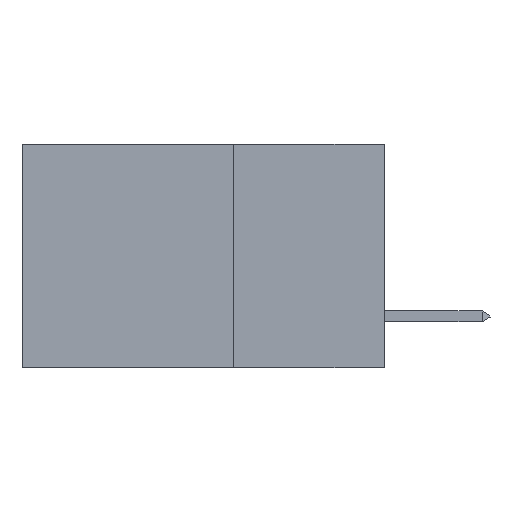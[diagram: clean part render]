
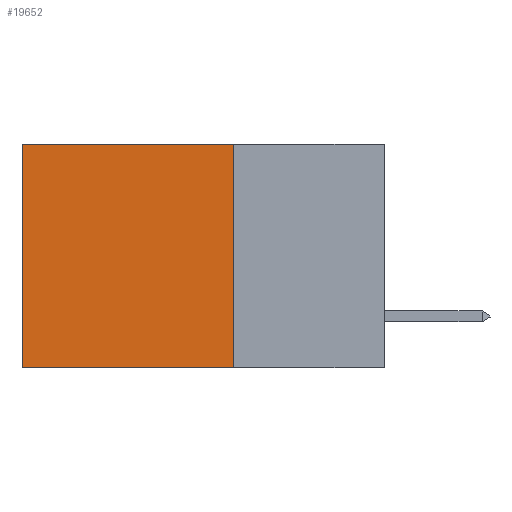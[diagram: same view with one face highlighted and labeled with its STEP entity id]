
A CAD part, left-side view. The second image highlights one B-rep face of the part: STEP entity #19652.
In plain terms, the highlighted planar face has unit normal (-1, 0, 0).
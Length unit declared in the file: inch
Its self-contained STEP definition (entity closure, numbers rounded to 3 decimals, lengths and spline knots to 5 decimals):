
#3214 = CARTESIAN_POINT ( 'NONE',  ( 0.2875, 0.25, 0. ) ) ;
#3326 = AXIS2_PLACEMENT_3D ( 'NONE', #8583, #22434, #37342 ) ;
#5509 = CARTESIAN_POINT ( 'NONE',  ( 0.2875, 0.25, -0.37 ) ) ;
#5762 = EDGE_CURVE ( 'NONE', #29457, #33184, #31142, .T. ) ;
#8160 = EDGE_CURVE ( 'NONE', #30288, #41633, #34900, .T. ) ;
#8583 = CARTESIAN_POINT ( 'NONE',  ( 0.2875, 0.25, 0. ) ) ;
#8875 = CARTESIAN_POINT ( 'NONE',  ( 0.2875, 0.25, 0. ) ) ;
#9150 = DIRECTION ( 'NONE',  ( 0., 1., 0. ) ) ;
#11128 = PLANE ( 'NONE',  #3326 ) ;
#11969 = LINE ( 'NONE', #22813, #42398 ) ;
#16475 = VECTOR ( 'NONE', #26170, 39.37008 ) ;
#19652 = ADVANCED_FACE ( 'NONE', ( #25178 ), #11128, .F. ) ;
#20322 = VECTOR ( 'NONE', #42332, 39.37008 ) ;
#20536 = CARTESIAN_POINT ( 'NONE',  ( 0.2875, 0.6, 0. ) ) ;
#21779 = ORIENTED_EDGE ( 'NONE', *, *, #8160, .F. ) ;
#22434 = DIRECTION ( 'NONE',  ( 1., 0., 0. ) ) ;
#22813 = CARTESIAN_POINT ( 'NONE',  ( 0.2875, 0.25, 0. ) ) ;
#25178 = FACE_OUTER_BOUND ( 'NONE', #35879, .T. ) ;
#25345 = VECTOR ( 'NONE', #9150, 39.37008 ) ;
#26170 = DIRECTION ( 'NONE',  ( 0., 1., 0. ) ) ;
#28706 = EDGE_CURVE ( 'NONE', #33184, #41633, #33818, .T. ) ;
#29457 = VERTEX_POINT ( 'NONE', #3214 ) ;
#30288 = VERTEX_POINT ( 'NONE', #37762 ) ;
#31142 = LINE ( 'NONE', #8875, #16475 ) ;
#33184 = VERTEX_POINT ( 'NONE', #36288 ) ;
#33818 = LINE ( 'NONE', #20536, #20322 ) ;
#34900 = LINE ( 'NONE', #5509, #25345 ) ;
#35879 = EDGE_LOOP ( 'NONE', ( #36474, #21779, #41128, #40969 ) ) ;
#36288 = CARTESIAN_POINT ( 'NONE',  ( 0.2875, 0.6, 0. ) ) ;
#36474 = ORIENTED_EDGE ( 'NONE', *, *, #28706, .T. ) ;
#37342 = DIRECTION ( 'NONE',  ( 0., 0., -1. ) ) ;
#37393 = DIRECTION ( 'NONE',  ( 0., 0., -1. ) ) ;
#37762 = CARTESIAN_POINT ( 'NONE',  ( 0.2875, 0.25, -0.37 ) ) ;
#40969 = ORIENTED_EDGE ( 'NONE', *, *, #5762, .T. ) ;
#41128 = ORIENTED_EDGE ( 'NONE', *, *, #42688, .F. ) ;
#41633 = VERTEX_POINT ( 'NONE', #45690 ) ;
#42332 = DIRECTION ( 'NONE',  ( 0., 0., -1. ) ) ;
#42398 = VECTOR ( 'NONE', #37393, 39.37008 ) ;
#42688 = EDGE_CURVE ( 'NONE', #29457, #30288, #11969, .T. ) ;
#45690 = CARTESIAN_POINT ( 'NONE',  ( 0.2875, 0.6, -0.37 ) ) ;
